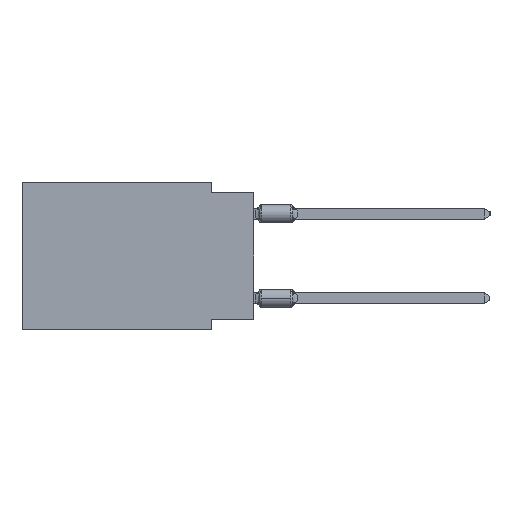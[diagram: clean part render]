
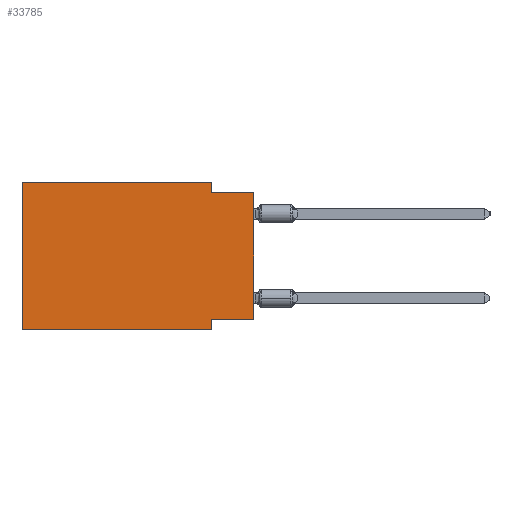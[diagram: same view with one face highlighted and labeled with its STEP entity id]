
A CAD part, left-side view. The second image highlights one B-rep face of the part: STEP entity #33785.
In plain terms, the highlighted planar face has unit normal (-1, 0, 0).
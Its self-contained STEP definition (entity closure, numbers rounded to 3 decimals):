
#531 = DIRECTION ( 'NONE',  ( 1., 0., 0. ) ) ;
#742 = CARTESIAN_POINT ( 'NONE',  ( 0., 13.97, 0. ) ) ;
#2661 = EDGE_CURVE ( 'NONE', #44172, #52954, #31759, .T. ) ;
#2843 = CARTESIAN_POINT ( 'NONE',  ( 0., 2.54, -8.89 ) ) ;
#4379 = PLANE ( 'NONE',  #52328 ) ;
#5579 = ORIENTED_EDGE ( 'NONE', *, *, #53722, .T. ) ;
#6898 = VECTOR ( 'NONE', #18749, 1000. ) ;
#7196 = VECTOR ( 'NONE', #28057, 1000. ) ;
#7538 = EDGE_CURVE ( 'NONE', #43658, #56947, #46148, .T. ) ;
#8324 = LINE ( 'NONE', #22475, #7196 ) ;
#9100 = DIRECTION ( 'NONE',  ( 0., 0., -1. ) ) ;
#10241 = CARTESIAN_POINT ( 'NONE',  ( 0., 0., -8.255 ) ) ;
#17329 = CARTESIAN_POINT ( 'NONE',  ( 0., 2.54, -8.89 ) ) ;
#17781 = VECTOR ( 'NONE', #33395, 1000. ) ;
#18652 = CARTESIAN_POINT ( 'NONE',  ( 0., 13.97, 0. ) ) ;
#18749 = DIRECTION ( 'NONE',  ( 0., -1., 0. ) ) ;
#19265 = LINE ( 'NONE', #37246, #17781 ) ;
#21275 = VERTEX_POINT ( 'NONE', #21573 ) ;
#21573 = CARTESIAN_POINT ( 'NONE',  ( 0., 0., -0.635 ) ) ;
#22356 = VECTOR ( 'NONE', #46794, 1000. ) ;
#22379 = CARTESIAN_POINT ( 'NONE',  ( 0., 13.97, 0. ) ) ;
#22475 = CARTESIAN_POINT ( 'NONE',  ( 0., 0., -0.635 ) ) ;
#24568 = VECTOR ( 'NONE', #35894, 1000. ) ;
#25353 = CARTESIAN_POINT ( 'NONE',  ( 0., 0., -8.255 ) ) ;
#27942 = EDGE_CURVE ( 'NONE', #45472, #44172, #54936, .T. ) ;
#28057 = DIRECTION ( 'NONE',  ( 0., -1., 0. ) ) ;
#28814 = LINE ( 'NONE', #56230, #22356 ) ;
#29473 = DIRECTION ( 'NONE',  ( 0., 1., 0. ) ) ;
#30558 = ORIENTED_EDGE ( 'NONE', *, *, #2661, .F. ) ;
#31759 = LINE ( 'NONE', #17329, #24568 ) ;
#32191 = CARTESIAN_POINT ( 'NONE',  ( 0., 2.54, -0.635 ) ) ;
#33395 = DIRECTION ( 'NONE',  ( 0., -1., 0. ) ) ;
#33785 = ADVANCED_FACE ( 'NONE', ( #53903 ), #4379, .F. ) ;
#33901 = CARTESIAN_POINT ( 'NONE',  ( 0., 0., 0. ) ) ;
#35894 = DIRECTION ( 'NONE',  ( 0., 0., -1. ) ) ;
#36488 = VERTEX_POINT ( 'NONE', #38352 ) ;
#37246 = CARTESIAN_POINT ( 'NONE',  ( 0., 13.97, -8.89 ) ) ;
#37652 = CARTESIAN_POINT ( 'NONE',  ( 0., 2.54, 0. ) ) ;
#38216 = EDGE_CURVE ( 'NONE', #45472, #21275, #57767, .T. ) ;
#38352 = CARTESIAN_POINT ( 'NONE',  ( 0., 13.97, -8.89 ) ) ;
#40035 = EDGE_LOOP ( 'NONE', ( #49849, #43297, #53213, #51866, #44985, #5579, #30558, #46841 ) ) ;
#43297 = ORIENTED_EDGE ( 'NONE', *, *, #56424, .F. ) ;
#43535 = VERTEX_POINT ( 'NONE', #32191 ) ;
#43658 = VERTEX_POINT ( 'NONE', #18652 ) ;
#44172 = VERTEX_POINT ( 'NONE', #46263 ) ;
#44985 = ORIENTED_EDGE ( 'NONE', *, *, #53446, .F. ) ;
#45472 = VERTEX_POINT ( 'NONE', #10241 ) ;
#46092 = VECTOR ( 'NONE', #52753, 1000. ) ;
#46148 = LINE ( 'NONE', #742, #6898 ) ;
#46263 = CARTESIAN_POINT ( 'NONE',  ( 0., 2.54, -8.255 ) ) ;
#46794 = DIRECTION ( 'NONE',  ( 0., 0., -1. ) ) ;
#46841 = ORIENTED_EDGE ( 'NONE', *, *, #27942, .F. ) ;
#48772 = CARTESIAN_POINT ( 'NONE',  ( 0., 13.97, 0. ) ) ;
#49849 = ORIENTED_EDGE ( 'NONE', *, *, #38216, .T. ) ;
#51866 = ORIENTED_EDGE ( 'NONE', *, *, #7538, .F. ) ;
#51883 = VECTOR ( 'NONE', #29473, 1000. ) ;
#52328 = AXIS2_PLACEMENT_3D ( 'NONE', #22379, #531, #9100 ) ;
#52753 = DIRECTION ( 'NONE',  ( 0., 0., 1. ) ) ;
#52877 = LINE ( 'NONE', #48772, #58215 ) ;
#52954 = VERTEX_POINT ( 'NONE', #2843 ) ;
#53213 = ORIENTED_EDGE ( 'NONE', *, *, #56948, .F. ) ;
#53446 = EDGE_CURVE ( 'NONE', #36488, #43658, #52877, .T. ) ;
#53722 = EDGE_CURVE ( 'NONE', #36488, #52954, #19265, .T. ) ;
#53903 = FACE_OUTER_BOUND ( 'NONE', #40035, .T. ) ;
#54936 = LINE ( 'NONE', #25353, #51883 ) ;
#56230 = CARTESIAN_POINT ( 'NONE',  ( 0., 2.54, 0. ) ) ;
#56424 = EDGE_CURVE ( 'NONE', #43535, #21275, #8324, .T. ) ;
#56947 = VERTEX_POINT ( 'NONE', #37652 ) ;
#56948 = EDGE_CURVE ( 'NONE', #56947, #43535, #28814, .T. ) ;
#57038 = DIRECTION ( 'NONE',  ( 0., 0., 1. ) ) ;
#57767 = LINE ( 'NONE', #33901, #46092 ) ;
#58215 = VECTOR ( 'NONE', #57038, 1000. ) ;
